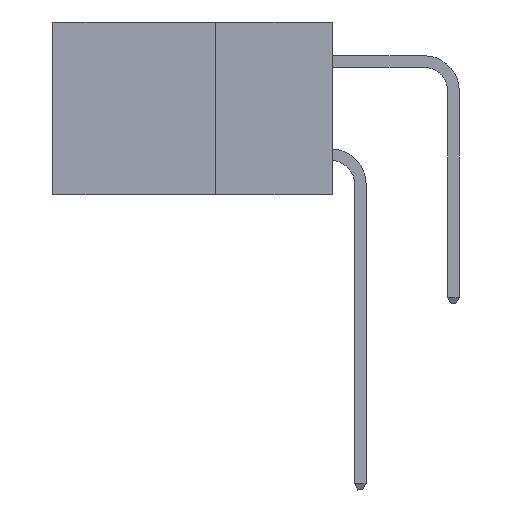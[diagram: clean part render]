
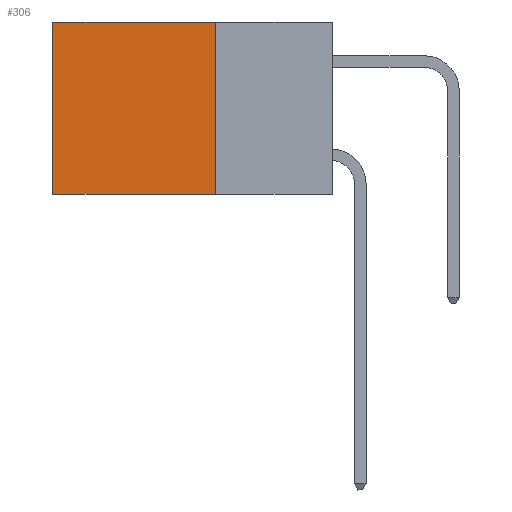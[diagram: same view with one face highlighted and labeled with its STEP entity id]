
A CAD part, left-side view. The second image highlights one B-rep face of the part: STEP entity #306.
In plain terms, the highlighted planar face has unit normal (-1, 0, 0).
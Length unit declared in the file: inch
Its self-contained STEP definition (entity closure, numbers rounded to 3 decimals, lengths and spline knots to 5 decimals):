
#306 = ADVANCED_FACE ( 'NONE', ( #6075 ), #3280, .F. ) ;
#1049 = CARTESIAN_POINT ( 'NONE',  ( 0.2615, 0.25, -0.37 ) ) ;
#2862 = EDGE_LOOP ( 'NONE', ( #23687, #6933, #7234, #14579 ) ) ;
#3280 = PLANE ( 'NONE',  #24756 ) ;
#3486 = CARTESIAN_POINT ( 'NONE',  ( 0.2615, 0.25, -0.37 ) ) ;
#4029 = CARTESIAN_POINT ( 'NONE',  ( 0.2615, 0.25, -0.37 ) ) ;
#6075 = FACE_OUTER_BOUND ( 'NONE', #2862, .T. ) ;
#6812 = VERTEX_POINT ( 'NONE', #13307 ) ;
#6933 = ORIENTED_EDGE ( 'NONE', *, *, #21037, .F. ) ;
#7234 = ORIENTED_EDGE ( 'NONE', *, *, #21892, .F. ) ;
#7379 = VECTOR ( 'NONE', #25262, 39.37008 ) ;
#7444 = VERTEX_POINT ( 'NONE', #15291 ) ;
#8177 = LINE ( 'NONE', #20898, #13924 ) ;
#9373 = VECTOR ( 'NONE', #10135, 39.37008 ) ;
#10018 = VECTOR ( 'NONE', #21462, 39.37008 ) ;
#10135 = DIRECTION ( 'NONE',  ( 0., 1., 0. ) ) ;
#13307 = CARTESIAN_POINT ( 'NONE',  ( 0.2615, 0.6, -0.37 ) ) ;
#13464 = VERTEX_POINT ( 'NONE', #14717 ) ;
#13827 = LINE ( 'NONE', #27551, #7379 ) ;
#13924 = VECTOR ( 'NONE', #16503, 39.37008 ) ;
#14579 = ORIENTED_EDGE ( 'NONE', *, *, #26376, .T. ) ;
#14717 = CARTESIAN_POINT ( 'NONE',  ( 0.2615, 0.25, 0. ) ) ;
#15291 = CARTESIAN_POINT ( 'NONE',  ( 0.2615, 0.6, 0. ) ) ;
#16503 = DIRECTION ( 'NONE',  ( 0., 1., 0. ) ) ;
#19772 = EDGE_CURVE ( 'NONE', #7444, #6812, #13827, .T. ) ;
#20898 = CARTESIAN_POINT ( 'NONE',  ( 0.2615, 0.25, 0. ) ) ;
#21037 = EDGE_CURVE ( 'NONE', #22343, #6812, #26693, .T. ) ;
#21462 = DIRECTION ( 'NONE',  ( 0., 0., -1. ) ) ;
#21892 = EDGE_CURVE ( 'NONE', #13464, #22343, #27329, .T. ) ;
#22343 = VERTEX_POINT ( 'NONE', #1049 ) ;
#22548 = CARTESIAN_POINT ( 'NONE',  ( 0.2615, 0.25, -0.37 ) ) ;
#23687 = ORIENTED_EDGE ( 'NONE', *, *, #19772, .T. ) ;
#24544 = DIRECTION ( 'NONE',  ( 1., 0., 0. ) ) ;
#24756 = AXIS2_PLACEMENT_3D ( 'NONE', #22548, #24544, #25181 ) ;
#25181 = DIRECTION ( 'NONE',  ( 0., 0., -1. ) ) ;
#25262 = DIRECTION ( 'NONE',  ( 0., 0., -1. ) ) ;
#26376 = EDGE_CURVE ( 'NONE', #13464, #7444, #8177, .T. ) ;
#26693 = LINE ( 'NONE', #3486, #9373 ) ;
#27329 = LINE ( 'NONE', #4029, #10018 ) ;
#27551 = CARTESIAN_POINT ( 'NONE',  ( 0.2615, 0.6, -0.37 ) ) ;
